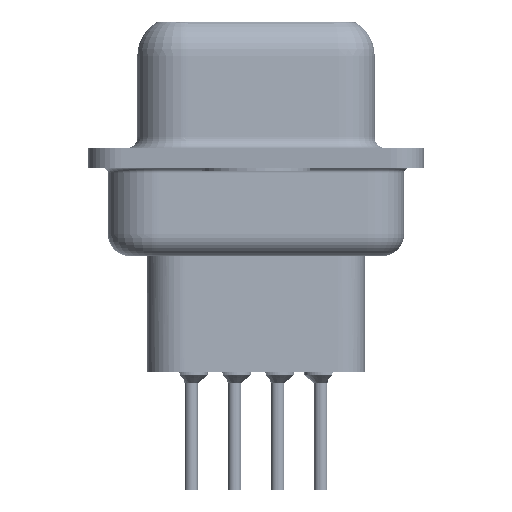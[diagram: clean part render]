
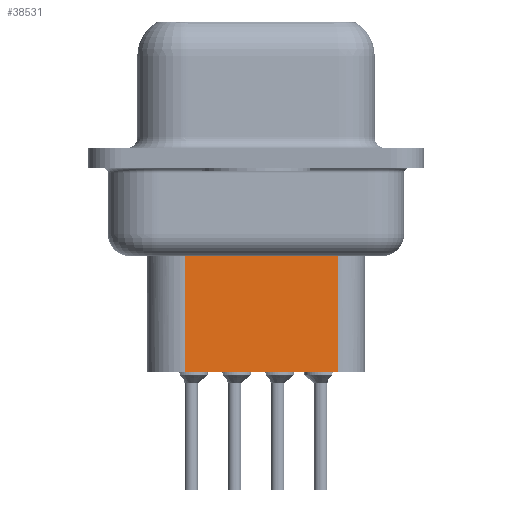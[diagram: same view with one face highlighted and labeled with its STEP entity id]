
A CAD part, left-side view. The second image highlights one B-rep face of the part: STEP entity #38531.
In plain terms, the highlighted planar face has unit normal (-0.985, -0.174, 0).
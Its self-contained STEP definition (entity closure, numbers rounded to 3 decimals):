
#780 = ORIENTED_EDGE ( 'NONE', *, *, #44595, .T. ) ;
#1073 = DIRECTION ( 'NONE',  ( -0.174, 0.985, 0. ) ) ;
#1563 = CARTESIAN_POINT ( 'NONE',  ( 4.624, 3.24, -9.85 ) ) ;
#1846 = LINE ( 'NONE', #3495, #52434 ) ;
#2097 = CARTESIAN_POINT ( 'NONE',  ( 4.624, 3.24, -3.975 ) ) ;
#2307 = AXIS2_PLACEMENT_3D ( 'NONE', #29934, #42369, #3632 ) ;
#2941 = CARTESIAN_POINT ( 'NONE',  ( 4.624, 3.24, -9.85 ) ) ;
#3495 = CARTESIAN_POINT ( 'NONE',  ( 4.624, 3.24, -3.1 ) ) ;
#3632 = DIRECTION ( 'NONE',  ( 0.174, -0.985, 0. ) ) ;
#4347 = LINE ( 'NONE', #5469, #12122 ) ;
#4435 = ORIENTED_EDGE ( 'NONE', *, *, #27938, .T. ) ;
#4640 = DIRECTION ( 'NONE',  ( 0., 0., -1. ) ) ;
#5469 = CARTESIAN_POINT ( 'NONE',  ( 5.858, -3.76, -3.1 ) ) ;
#5805 = VECTOR ( 'NONE', #19629, 1000. ) ;
#8199 = ORIENTED_EDGE ( 'NONE', *, *, #54774, .F. ) ;
#8735 = VERTEX_POINT ( 'NONE', #48776 ) ;
#12122 = VECTOR ( 'NONE', #4640, 1000. ) ;
#13257 = VECTOR ( 'NONE', #1073, 1000. ) ;
#15844 = CARTESIAN_POINT ( 'NONE',  ( 5.858, -3.76, -3.975 ) ) ;
#16185 = EDGE_CURVE ( 'NONE', #46670, #8735, #4347, .T. ) ;
#19031 = VERTEX_POINT ( 'NONE', #2097 ) ;
#19629 = DIRECTION ( 'NONE',  ( -0.174, 0.985, 0. ) ) ;
#20891 = PLANE ( 'NONE',  #2307 ) ;
#25416 = FACE_OUTER_BOUND ( 'NONE', #42617, .T. ) ;
#25521 = ORIENTED_EDGE ( 'NONE', *, *, #16185, .F. ) ;
#27342 = CARTESIAN_POINT ( 'NONE',  ( 4.453, 4.209, -3.975 ) ) ;
#27938 = EDGE_CURVE ( 'NONE', #46670, #19031, #40352, .T. ) ;
#29934 = CARTESIAN_POINT ( 'NONE',  ( 4.624, 3.24, -3.1 ) ) ;
#32149 = VERTEX_POINT ( 'NONE', #2941 ) ;
#37190 = DIRECTION ( 'NONE',  ( 0., 0., -1. ) ) ;
#38531 = ADVANCED_FACE ( 'NONE', ( #25416 ), #20891, .T. ) ;
#40352 = LINE ( 'NONE', #27342, #13257 ) ;
#42369 = DIRECTION ( 'NONE',  ( -0.985, -0.174, 0. ) ) ;
#42617 = EDGE_LOOP ( 'NONE', ( #25521, #4435, #780, #8199 ) ) ;
#44595 = EDGE_CURVE ( 'NONE', #19031, #32149, #1846, .T. ) ;
#46670 = VERTEX_POINT ( 'NONE', #15844 ) ;
#48776 = CARTESIAN_POINT ( 'NONE',  ( 5.858, -3.76, -9.85 ) ) ;
#49300 = LINE ( 'NONE', #1563, #5805 ) ;
#52434 = VECTOR ( 'NONE', #37190, 1000. ) ;
#54774 = EDGE_CURVE ( 'NONE', #8735, #32149, #49300, .T. ) ;
